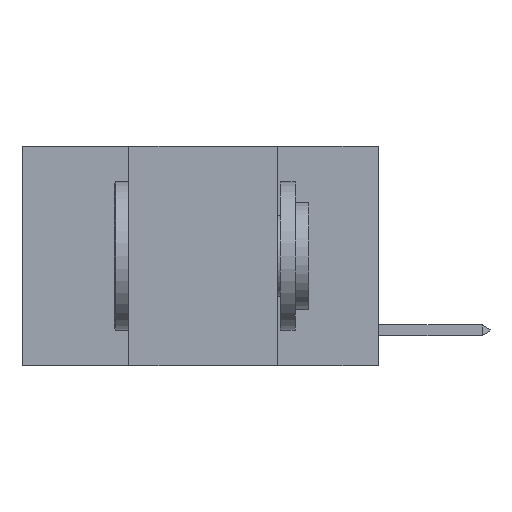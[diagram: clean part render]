
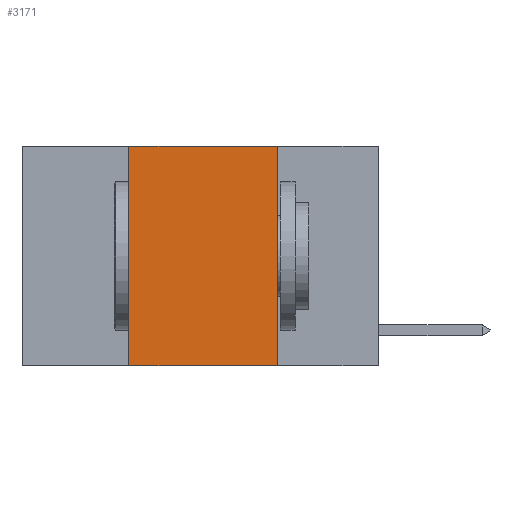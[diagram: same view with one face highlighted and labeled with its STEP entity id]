
A CAD part, left-side view. The second image highlights one B-rep face of the part: STEP entity #3171.
In plain terms, the highlighted planar face has unit normal (-1, 0, 0).
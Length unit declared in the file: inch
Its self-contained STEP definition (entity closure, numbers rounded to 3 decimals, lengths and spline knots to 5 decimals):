
#603 = CARTESIAN_POINT ( 'NONE',  ( 0., 0.6, 0. ) ) ;
#830 = VECTOR ( 'NONE', #19341, 39.37008 ) ;
#1207 = CARTESIAN_POINT ( 'NONE',  ( 0., 0.6, 0. ) ) ;
#2392 = CARTESIAN_POINT ( 'NONE',  ( 0., 0.42, -0.37 ) ) ;
#2614 = VECTOR ( 'NONE', #19580, 39.37008 ) ;
#3171 = ADVANCED_FACE ( 'NONE', ( #18512 ), #11747, .F. ) ;
#4360 = CARTESIAN_POINT ( 'NONE',  ( 0., 0.17, 0. ) ) ;
#4539 = CARTESIAN_POINT ( 'NONE',  ( 0., 0.42, 0. ) ) ;
#4678 = LINE ( 'NONE', #4539, #830 ) ;
#5121 = AXIS2_PLACEMENT_3D ( 'NONE', #1207, #10088, #18096 ) ;
#5233 = ORIENTED_EDGE ( 'NONE', *, *, #12457, .T. ) ;
#6103 = DIRECTION ( 'NONE',  ( 0., -1., 0. ) ) ;
#7398 = DIRECTION ( 'NONE',  ( 0., -1., 0. ) ) ;
#7596 = VECTOR ( 'NONE', #6103, 39.37008 ) ;
#8345 = VERTEX_POINT ( 'NONE', #16460 ) ;
#10088 = DIRECTION ( 'NONE',  ( 1., 0., 0. ) ) ;
#10179 = ORIENTED_EDGE ( 'NONE', *, *, #15322, .F. ) ;
#11747 = PLANE ( 'NONE',  #5121 ) ;
#12119 = VECTOR ( 'NONE', #7398, 39.37008 ) ;
#12258 = EDGE_LOOP ( 'NONE', ( #17010, #22680, #10179, #5233 ) ) ;
#12457 = EDGE_CURVE ( 'NONE', #17675, #14963, #27162, .T. ) ;
#13909 = LINE ( 'NONE', #603, #12119 ) ;
#14594 = EDGE_CURVE ( 'NONE', #23580, #14963, #25695, .T. ) ;
#14963 = VERTEX_POINT ( 'NONE', #26656 ) ;
#15322 = EDGE_CURVE ( 'NONE', #17675, #8345, #4678, .T. ) ;
#16460 = CARTESIAN_POINT ( 'NONE',  ( 0., 0.42, 0. ) ) ;
#17010 = ORIENTED_EDGE ( 'NONE', *, *, #14594, .F. ) ;
#17675 = VERTEX_POINT ( 'NONE', #2392 ) ;
#18096 = DIRECTION ( 'NONE',  ( 0., 0., -1. ) ) ;
#18512 = FACE_OUTER_BOUND ( 'NONE', #12258, .T. ) ;
#19341 = DIRECTION ( 'NONE',  ( 0., 0., 1. ) ) ;
#19580 = DIRECTION ( 'NONE',  ( 0., 0., -1. ) ) ;
#20513 = CARTESIAN_POINT ( 'NONE',  ( 0., 0.6, -0.37 ) ) ;
#22680 = ORIENTED_EDGE ( 'NONE', *, *, #25912, .F. ) ;
#23580 = VERTEX_POINT ( 'NONE', #24235 ) ;
#24235 = CARTESIAN_POINT ( 'NONE',  ( 0., 0.17, 0. ) ) ;
#25695 = LINE ( 'NONE', #4360, #2614 ) ;
#25912 = EDGE_CURVE ( 'NONE', #8345, #23580, #13909, .T. ) ;
#26656 = CARTESIAN_POINT ( 'NONE',  ( 0., 0.17, -0.37 ) ) ;
#27162 = LINE ( 'NONE', #20513, #7596 ) ;
